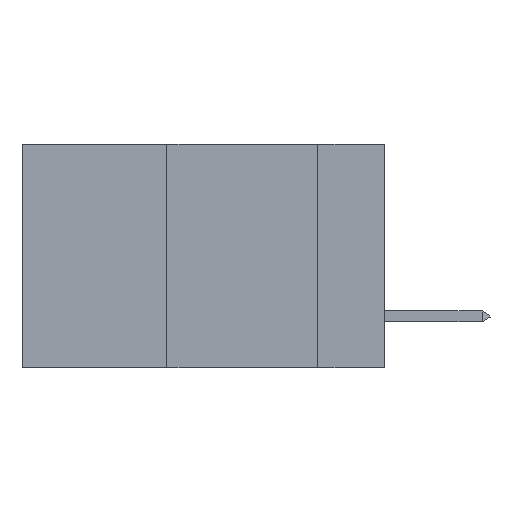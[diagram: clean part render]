
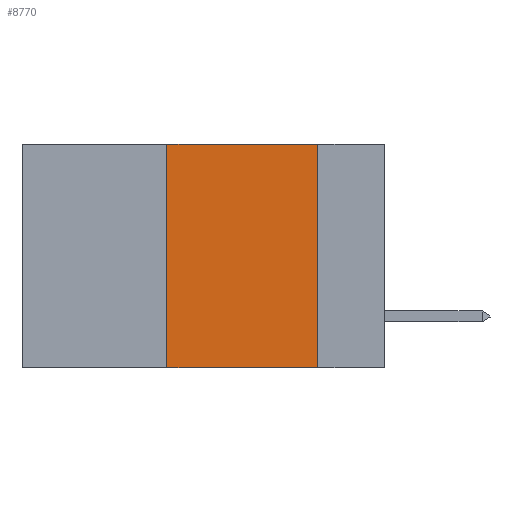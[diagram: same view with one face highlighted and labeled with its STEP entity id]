
A CAD part, left-side view. The second image highlights one B-rep face of the part: STEP entity #8770.
In plain terms, the highlighted planar face has unit normal (-1, 0, 0).
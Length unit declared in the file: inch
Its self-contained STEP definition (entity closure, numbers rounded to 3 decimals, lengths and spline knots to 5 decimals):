
#98 = VERTEX_POINT ( 'NONE', #153 ) ;
#153 = CARTESIAN_POINT ( 'NONE',  ( 0., 0.11, 0. ) ) ;
#355 = CARTESIAN_POINT ( 'NONE',  ( 0., 0.36, -0.37 ) ) ;
#488 = EDGE_CURVE ( 'NONE', #4561, #98, #1618, .T. ) ;
#506 = VECTOR ( 'NONE', #6212, 39.37008 ) ;
#520 = CARTESIAN_POINT ( 'NONE',  ( 0., 0.6, 0. ) ) ;
#1563 = LINE ( 'NONE', #5917, #10729 ) ;
#1618 = LINE ( 'NONE', #5546, #7158 ) ;
#2842 = CARTESIAN_POINT ( 'NONE',  ( 0., 0.36, 0. ) ) ;
#3057 = ORIENTED_EDGE ( 'NONE', *, *, #7942, .F. ) ;
#3408 = PLANE ( 'NONE',  #4741 ) ;
#3560 = EDGE_CURVE ( 'NONE', #98, #11665, #1563, .T. ) ;
#3664 = CARTESIAN_POINT ( 'NONE',  ( 0., 0.11, -0.37 ) ) ;
#4561 = VERTEX_POINT ( 'NONE', #5279 ) ;
#4741 = AXIS2_PLACEMENT_3D ( 'NONE', #520, #6996, #5486 ) ;
#5279 = CARTESIAN_POINT ( 'NONE',  ( 0., 0.36, 0. ) ) ;
#5486 = DIRECTION ( 'NONE',  ( 0., 0., -1. ) ) ;
#5498 = EDGE_LOOP ( 'NONE', ( #7274, #11167, #3057, #7464 ) ) ;
#5546 = CARTESIAN_POINT ( 'NONE',  ( 0., 0.6, 0. ) ) ;
#5917 = CARTESIAN_POINT ( 'NONE',  ( 0., 0.11, 0. ) ) ;
#6212 = DIRECTION ( 'NONE',  ( 0., -1., 0. ) ) ;
#6996 = DIRECTION ( 'NONE',  ( 1., 0., 0. ) ) ;
#7158 = VECTOR ( 'NONE', #7554, 39.37008 ) ;
#7274 = ORIENTED_EDGE ( 'NONE', *, *, #3560, .F. ) ;
#7281 = VERTEX_POINT ( 'NONE', #355 ) ;
#7464 = ORIENTED_EDGE ( 'NONE', *, *, #11655, .T. ) ;
#7466 = LINE ( 'NONE', #2842, #9822 ) ;
#7554 = DIRECTION ( 'NONE',  ( 0., -1., 0. ) ) ;
#7706 = DIRECTION ( 'NONE',  ( 0., 0., -1. ) ) ;
#7942 = EDGE_CURVE ( 'NONE', #7281, #4561, #7466, .T. ) ;
#8770 = ADVANCED_FACE ( 'NONE', ( #11687 ), #3408, .F. ) ;
#9525 = DIRECTION ( 'NONE',  ( 0., 0., 1. ) ) ;
#9822 = VECTOR ( 'NONE', #9525, 39.37008 ) ;
#10300 = LINE ( 'NONE', #10792, #506 ) ;
#10729 = VECTOR ( 'NONE', #7706, 39.37008 ) ;
#10792 = CARTESIAN_POINT ( 'NONE',  ( 0., 0.6, -0.37 ) ) ;
#11167 = ORIENTED_EDGE ( 'NONE', *, *, #488, .F. ) ;
#11655 = EDGE_CURVE ( 'NONE', #7281, #11665, #10300, .T. ) ;
#11665 = VERTEX_POINT ( 'NONE', #3664 ) ;
#11687 = FACE_OUTER_BOUND ( 'NONE', #5498, .T. ) ;
